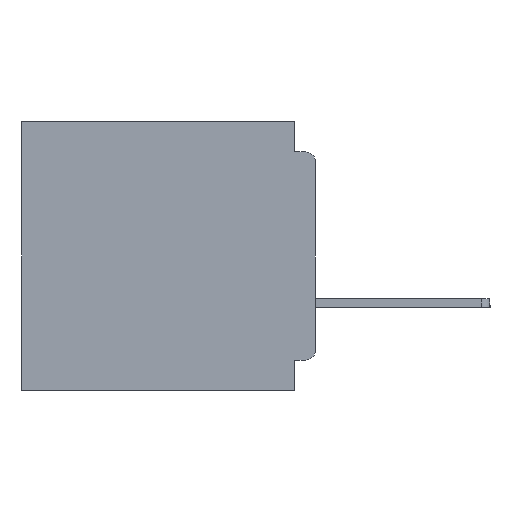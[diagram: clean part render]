
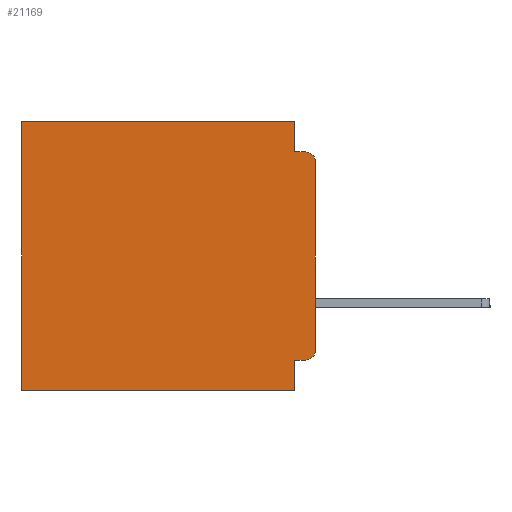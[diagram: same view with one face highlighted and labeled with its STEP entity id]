
A CAD part, left-side view. The second image highlights one B-rep face of the part: STEP entity #21169.
In plain terms, the highlighted planar face has unit normal (-1, 0, 0).
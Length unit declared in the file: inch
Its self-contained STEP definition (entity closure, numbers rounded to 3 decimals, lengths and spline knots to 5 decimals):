
#63 = DIRECTION ( 'NONE',  ( 0., 0., -1. ) ) ;
#105 = ORIENTED_EDGE ( 'NONE', *, *, #39662, .F. ) ;
#212 = CARTESIAN_POINT ( 'NONE',  ( 0.3, 0.031, -0.4 ) ) ;
#549 = CARTESIAN_POINT ( 'NONE',  ( 0.3, 0.031, 0. ) ) ;
#639 = ORIENTED_EDGE ( 'NONE', *, *, #11158, .F. ) ;
#896 = EDGE_CURVE ( 'NONE', #20685, #24079, #27583, .T. ) ;
#990 = ORIENTED_EDGE ( 'NONE', *, *, #896, .T. ) ;
#1155 = ORIENTED_EDGE ( 'NONE', *, *, #29001, .T. ) ;
#1511 = VECTOR ( 'NONE', #16259, 39.37008 ) ;
#1604 = ORIENTED_EDGE ( 'NONE', *, *, #18537, .F. ) ;
#1657 = CARTESIAN_POINT ( 'NONE',  ( 0.3, 0., 0. ) ) ;
#1672 = ORIENTED_EDGE ( 'NONE', *, *, #31227, .F. ) ;
#1945 = ORIENTED_EDGE ( 'NONE', *, *, #31053, .F. ) ;
#2105 = ORIENTED_EDGE ( 'NONE', *, *, #6401, .T. ) ;
#2433 = VERTEX_POINT ( 'NONE', #19836 ) ;
#4073 = CARTESIAN_POINT ( 'NONE',  ( 0.3, 0., -0.355 ) ) ;
#5938 = CARTESIAN_POINT ( 'NONE',  ( 0.3, 0.031, 0. ) ) ;
#6118 = DIRECTION ( 'NONE',  ( -1., 0., 0. ) ) ;
#6401 = EDGE_CURVE ( 'NONE', #29900, #25476, #27877, .T. ) ;
#6768 = EDGE_CURVE ( 'NONE', #13608, #40020, #39220, .T. ) ;
#7352 = CARTESIAN_POINT ( 'NONE',  ( 0.3, 0.437, 0. ) ) ;
#8584 = VECTOR ( 'NONE', #31866, 39.37008 ) ;
#9469 = CARTESIAN_POINT ( 'NONE',  ( 0.3, 0., -0.06 ) ) ;
#10780 = CARTESIAN_POINT ( 'NONE',  ( 0.3, 0.015, -0.34 ) ) ;
#10962 = DIRECTION ( 'NONE',  ( 0., 0., -1. ) ) ;
#11158 = EDGE_CURVE ( 'NONE', #20685, #2433, #17403, .T. ) ;
#11714 = CARTESIAN_POINT ( 'NONE',  ( 0.3, 0.031, -0.4 ) ) ;
#11799 = VECTOR ( 'NONE', #39514, 39.37008 ) ;
#12924 = VECTOR ( 'NONE', #28251, 39.37008 ) ;
#13608 = VERTEX_POINT ( 'NONE', #9469 ) ;
#13696 = VERTEX_POINT ( 'NONE', #212 ) ;
#13839 = LINE ( 'NONE', #4073, #29958 ) ;
#14104 = DIRECTION ( 'NONE',  ( 0., 0., -1. ) ) ;
#14293 = CARTESIAN_POINT ( 'NONE',  ( 0.3, 0.437, -0.4 ) ) ;
#14332 = VECTOR ( 'NONE', #15034, 39.37008 ) ;
#15034 = DIRECTION ( 'NONE',  ( 0., 0., -1. ) ) ;
#16058 = CARTESIAN_POINT ( 'NONE',  ( 0.3, 0.437, -0.4 ) ) ;
#16259 = DIRECTION ( 'NONE',  ( 0., 1., 0. ) ) ;
#16314 = FACE_OUTER_BOUND ( 'NONE', #23100, .T. ) ;
#16331 = VECTOR ( 'NONE', #27539, 39.37008 ) ;
#16413 = LINE ( 'NONE', #11714, #14332 ) ;
#16569 = CARTESIAN_POINT ( 'NONE',  ( 0.3, 0.015, -0.045 ) ) ;
#16582 = PLANE ( 'NONE',  #29784 ) ;
#16791 = LINE ( 'NONE', #14293, #41144 ) ;
#17367 = LINE ( 'NONE', #24370, #16331 ) ;
#17403 = LINE ( 'NONE', #5938, #8584 ) ;
#18537 = EDGE_CURVE ( 'NONE', #13696, #26902, #21625, .T. ) ;
#19836 = CARTESIAN_POINT ( 'NONE',  ( 0.3, 0.031, -0.045 ) ) ;
#19847 = DIRECTION ( 'NONE',  ( 1., 0., 0. ) ) ;
#20685 = VERTEX_POINT ( 'NONE', #549 ) ;
#21169 = ADVANCED_FACE ( 'NONE', ( #16314 ), #16582, .F. ) ;
#21625 = LINE ( 'NONE', #40823, #12924 ) ;
#23100 = EDGE_LOOP ( 'NONE', ( #25382, #38905, #105, #639, #990, #1155, #1604, #1672, #1945, #2105 ) ) ;
#24079 = VERTEX_POINT ( 'NONE', #7352 ) ;
#24370 = CARTESIAN_POINT ( 'NONE',  ( 0.3, 0., -0.045 ) ) ;
#25382 = ORIENTED_EDGE ( 'NONE', *, *, #38294, .F. ) ;
#25476 = VERTEX_POINT ( 'NONE', #27475 ) ;
#25477 = AXIS2_PLACEMENT_3D ( 'NONE', #10780, #33299, #14104 ) ;
#25691 = CARTESIAN_POINT ( 'NONE',  ( 0.3, 0.015, -0.06 ) ) ;
#26902 = VERTEX_POINT ( 'NONE', #16058 ) ;
#27475 = CARTESIAN_POINT ( 'NONE',  ( 0.3, 0., -0.34 ) ) ;
#27539 = DIRECTION ( 'NONE',  ( 0., -1., 0. ) ) ;
#27583 = LINE ( 'NONE', #1657, #1511 ) ;
#27877 = CIRCLE ( 'NONE', #25477, 0.015 ) ;
#28251 = DIRECTION ( 'NONE',  ( 0., 1., 0. ) ) ;
#28878 = DIRECTION ( 'NONE',  ( 0., 0., -1. ) ) ;
#29001 = EDGE_CURVE ( 'NONE', #24079, #26902, #16791, .T. ) ;
#29753 = CARTESIAN_POINT ( 'NONE',  ( 0.3, 0.015, -0.355 ) ) ;
#29784 = AXIS2_PLACEMENT_3D ( 'NONE', #38832, #19847, #63 ) ;
#29900 = VERTEX_POINT ( 'NONE', #29753 ) ;
#29958 = VECTOR ( 'NONE', #33105, 39.37008 ) ;
#31053 = EDGE_CURVE ( 'NONE', #29900, #39260, #13839, .T. ) ;
#31227 = EDGE_CURVE ( 'NONE', #39260, #13696, #16413, .T. ) ;
#31866 = DIRECTION ( 'NONE',  ( 0., 0., -1. ) ) ;
#33105 = DIRECTION ( 'NONE',  ( 0., 1., 0. ) ) ;
#33299 = DIRECTION ( 'NONE',  ( -1., 0., 0. ) ) ;
#36338 = CARTESIAN_POINT ( 'NONE',  ( 0.3, 0., -0.4 ) ) ;
#37368 = LINE ( 'NONE', #36338, #11799 ) ;
#37371 = AXIS2_PLACEMENT_3D ( 'NONE', #25691, #6118, #28878 ) ;
#38022 = CARTESIAN_POINT ( 'NONE',  ( 0.3, 0.031, -0.355 ) ) ;
#38294 = EDGE_CURVE ( 'NONE', #13608, #25476, #37368, .T. ) ;
#38832 = CARTESIAN_POINT ( 'NONE',  ( 0.3, 0., -0.4 ) ) ;
#38905 = ORIENTED_EDGE ( 'NONE', *, *, #6768, .T. ) ;
#39220 = CIRCLE ( 'NONE', #37371, 0.015 ) ;
#39260 = VERTEX_POINT ( 'NONE', #38022 ) ;
#39514 = DIRECTION ( 'NONE',  ( 0., 0., -1. ) ) ;
#39662 = EDGE_CURVE ( 'NONE', #2433, #40020, #17367, .T. ) ;
#40020 = VERTEX_POINT ( 'NONE', #16569 ) ;
#40823 = CARTESIAN_POINT ( 'NONE',  ( 0.3, 0., -0.4 ) ) ;
#41144 = VECTOR ( 'NONE', #10962, 39.37008 ) ;
